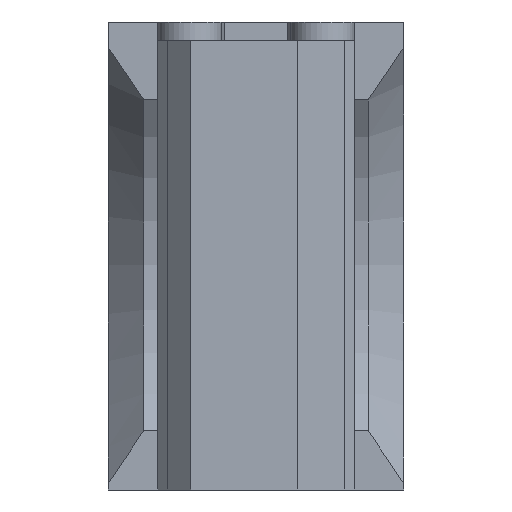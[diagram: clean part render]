
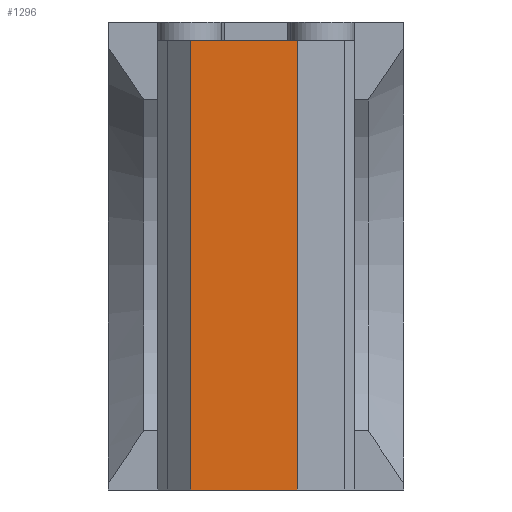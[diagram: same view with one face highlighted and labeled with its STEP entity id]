
A CAD part, left-side view. The second image highlights one B-rep face of the part: STEP entity #1296.
In plain terms, the highlighted planar face has unit normal (-1, 0, 0).
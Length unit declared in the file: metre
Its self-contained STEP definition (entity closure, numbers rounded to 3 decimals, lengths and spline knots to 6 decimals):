
#26=PLANE('',#1404);
#123=LINE('',#2018,#270);
#156=LINE('',#2092,#303);
#171=LINE('',#2121,#318);
#172=LINE('',#2122,#319);
#270=VECTOR('',#1584,1.);
#303=VECTOR('',#1637,1.);
#318=VECTOR('',#1662,1.);
#319=VECTOR('',#1663,1.);
#546=ORIENTED_EDGE('',*,*,#882,.T.);
#547=ORIENTED_EDGE('',*,*,#900,.T.);
#548=ORIENTED_EDGE('',*,*,#841,.F.);
#549=ORIENTED_EDGE('',*,*,#901,.T.);
#841=EDGE_CURVE('',#1021,#1022,#123,.T.);
#882=EDGE_CURVE('',#1053,#1052,#156,.T.);
#900=EDGE_CURVE('',#1052,#1022,#171,.T.);
#901=EDGE_CURVE('',#1021,#1053,#172,.T.);
#1021=VERTEX_POINT('',#2017);
#1022=VERTEX_POINT('',#2019);
#1052=VERTEX_POINT('',#2091);
#1053=VERTEX_POINT('',#2093);
#1134=EDGE_LOOP('',(#546,#547,#548,#549));
#1213=FACE_BOUND('',#1134,.T.);
#1296=ADVANCED_FACE('',(#1213),#26,.T.);
#1404=AXIS2_PLACEMENT_3D('',#2120,#1660,#1661);
#1584=DIRECTION('',(0.,-1.,0.));
#1637=DIRECTION('',(0.,-1.,0.));
#1660=DIRECTION('',(-1.,0.,0.));
#1661=DIRECTION('',(0.,0.,1.));
#1662=DIRECTION('',(0.,0.,1.));
#1663=DIRECTION('',(0.,0.,-1.));
#2017=CARTESIAN_POINT('',(-0.057277,0.003493,0.021463));
#2018=CARTESIAN_POINT('',(-0.057277,0.,0.021463));
#2019=CARTESIAN_POINT('',(-0.057277,-0.002223,0.021463));
#2091=CARTESIAN_POINT('',(-0.057277,-0.002223,-0.002667));
#2092=CARTESIAN_POINT('',(-0.057277,0.,-0.002667));
#2093=CARTESIAN_POINT('',(-0.057277,0.003493,-0.002667));
#2120=CARTESIAN_POINT('',(-0.057277,0.,0.009398));
#2121=CARTESIAN_POINT('',(-0.057277,-0.002223,0.009398));
#2122=CARTESIAN_POINT('',(-0.057277,0.003493,-0.002667));
